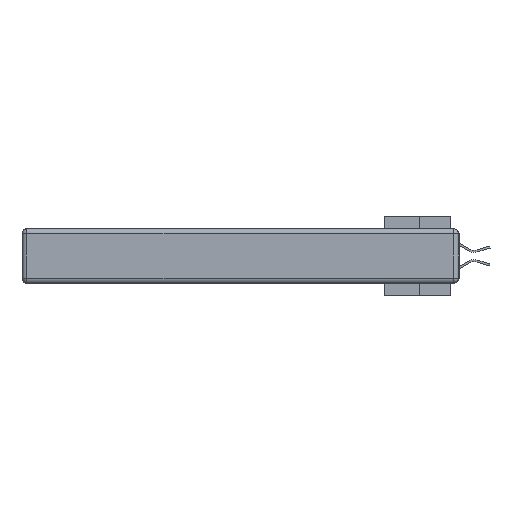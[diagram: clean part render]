
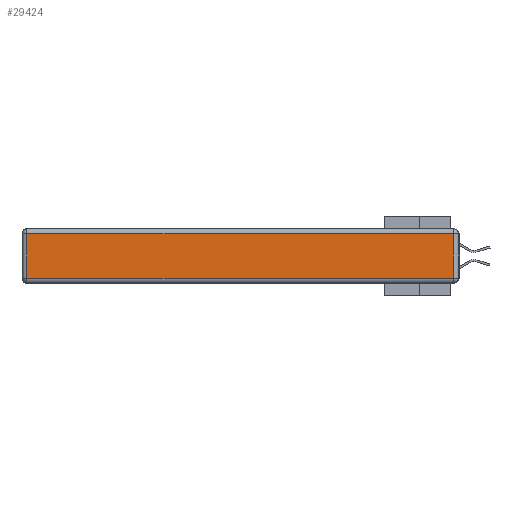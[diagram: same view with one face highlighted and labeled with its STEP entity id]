
A CAD part, left-side view. The second image highlights one B-rep face of the part: STEP entity #29424.
In plain terms, the highlighted planar face has unit normal (-1, 0, 0).
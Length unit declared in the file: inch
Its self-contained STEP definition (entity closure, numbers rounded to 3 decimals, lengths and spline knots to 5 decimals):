
#316 = CARTESIAN_POINT ( 'NONE',  ( 0., 0.03, -0.03 ) ) ;
#518 = CARTESIAN_POINT ( 'NONE',  ( 0., 0., -0.343 ) ) ;
#2266 = CARTESIAN_POINT ( 'NONE',  ( 0., 0.03, -0.313 ) ) ;
#2434 = ORIENTED_EDGE ( 'NONE', *, *, #19551, .T. ) ;
#3971 = ORIENTED_EDGE ( 'NONE', *, *, #22506, .T. ) ;
#3985 = LINE ( 'NONE', #25638, #29334 ) ;
#4013 = CARTESIAN_POINT ( 'NONE',  ( 0., 2.72, -0.03 ) ) ;
#6145 = EDGE_CURVE ( 'NONE', #10409, #7055, #22447, .T. ) ;
#7055 = VERTEX_POINT ( 'NONE', #4013 ) ;
#8295 = ORIENTED_EDGE ( 'NONE', *, *, #23475, .T. ) ;
#8548 = CARTESIAN_POINT ( 'NONE',  ( 0., 2.72, -0.313 ) ) ;
#9065 = EDGE_LOOP ( 'NONE', ( #8295, #3971, #11343, #2434 ) ) ;
#9887 = VECTOR ( 'NONE', #25201, 39.37008 ) ;
#10409 = VERTEX_POINT ( 'NONE', #316 ) ;
#11074 = AXIS2_PLACEMENT_3D ( 'NONE', #518, #26271, #28798 ) ;
#11343 = ORIENTED_EDGE ( 'NONE', *, *, #6145, .T. ) ;
#14670 = DIRECTION ( 'NONE',  ( 0., 0., 1. ) ) ;
#15539 = CARTESIAN_POINT ( 'NONE',  ( 0., 2.75, -0.03 ) ) ;
#15635 = LINE ( 'NONE', #22702, #9887 ) ;
#15744 = DIRECTION ( 'NONE',  ( 0., 0., -1. ) ) ;
#17029 = PLANE ( 'NONE',  #11074 ) ;
#17032 = CARTESIAN_POINT ( 'NONE',  ( 0., 0.03, -0.343 ) ) ;
#18210 = DIRECTION ( 'NONE',  ( 0., 1., 0. ) ) ;
#18876 = VECTOR ( 'NONE', #14670, 39.37008 ) ;
#19551 = EDGE_CURVE ( 'NONE', #7055, #19579, #3985, .T. ) ;
#19579 = VERTEX_POINT ( 'NONE', #8548 ) ;
#22060 = FACE_OUTER_BOUND ( 'NONE', #9065, .T. ) ;
#22447 = LINE ( 'NONE', #15539, #25377 ) ;
#22506 = EDGE_CURVE ( 'NONE', #24914, #10409, #24411, .T. ) ;
#22702 = CARTESIAN_POINT ( 'NONE',  ( 0., 0., -0.313 ) ) ;
#23475 = EDGE_CURVE ( 'NONE', #19579, #24914, #15635, .T. ) ;
#24411 = LINE ( 'NONE', #17032, #18876 ) ;
#24914 = VERTEX_POINT ( 'NONE', #2266 ) ;
#25201 = DIRECTION ( 'NONE',  ( 0., -1., 0. ) ) ;
#25377 = VECTOR ( 'NONE', #18210, 39.37008 ) ;
#25638 = CARTESIAN_POINT ( 'NONE',  ( 0., 2.72, -0.343 ) ) ;
#26271 = DIRECTION ( 'NONE',  ( -1., 0., 0. ) ) ;
#28798 = DIRECTION ( 'NONE',  ( 0., 0., 1. ) ) ;
#29334 = VECTOR ( 'NONE', #15744, 39.37008 ) ;
#29424 = ADVANCED_FACE ( 'NONE', ( #22060 ), #17029, .T. ) ;
